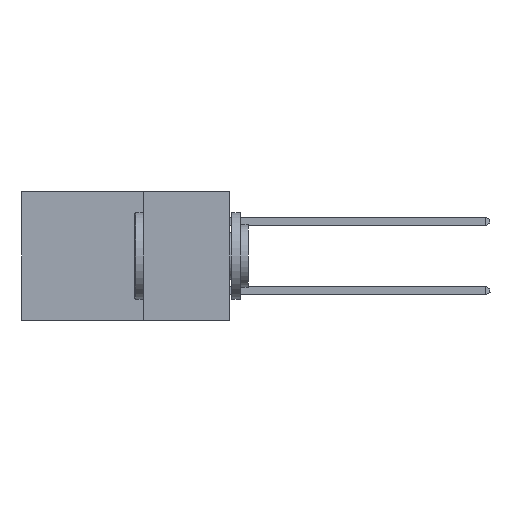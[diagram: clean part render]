
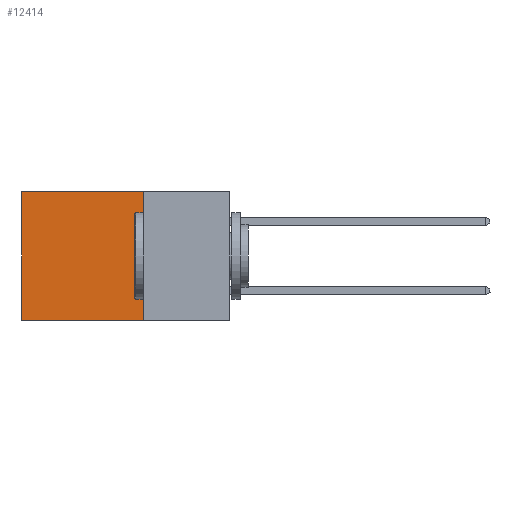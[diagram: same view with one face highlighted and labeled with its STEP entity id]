
A CAD part, left-side view. The second image highlights one B-rep face of the part: STEP entity #12414.
In plain terms, the highlighted planar face has unit normal (-1, 0, 0).
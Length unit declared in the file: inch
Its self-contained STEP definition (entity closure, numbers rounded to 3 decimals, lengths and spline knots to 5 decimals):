
#145 = AXIS2_PLACEMENT_3D ( 'NONE', #27502, #13374, #29830 ) ;
#390 = DIRECTION ( 'NONE',  ( 0., 1., 0. ) ) ;
#1108 = ORIENTED_EDGE ( 'NONE', *, *, #8051, .F. ) ;
#1260 = CARTESIAN_POINT ( 'NONE',  ( 0.298, 0.25, -0.37 ) ) ;
#1851 = CARTESIAN_POINT ( 'NONE',  ( 0.298, 0.25, -0.37 ) ) ;
#2516 = LINE ( 'NONE', #3339, #26216 ) ;
#2704 = VECTOR ( 'NONE', #30235, 39.37008 ) ;
#3339 = CARTESIAN_POINT ( 'NONE',  ( 0.298, 0.25, 0. ) ) ;
#3386 = FACE_OUTER_BOUND ( 'NONE', #28987, .T. ) ;
#5397 = CARTESIAN_POINT ( 'NONE',  ( 0.298, 0.6, 0. ) ) ;
#7564 = EDGE_CURVE ( 'NONE', #11516, #7725, #20928, .T. ) ;
#7725 = VERTEX_POINT ( 'NONE', #16689 ) ;
#8051 = EDGE_CURVE ( 'NONE', #11173, #20440, #2516, .T. ) ;
#8615 = PLANE ( 'NONE',  #145 ) ;
#10556 = DIRECTION ( 'NONE',  ( 0., 0., -1. ) ) ;
#10692 = EDGE_CURVE ( 'NONE', #11173, #11516, #22455, .T. ) ;
#11173 = VERTEX_POINT ( 'NONE', #16038 ) ;
#11516 = VERTEX_POINT ( 'NONE', #5397 ) ;
#12100 = LINE ( 'NONE', #1851, #27944 ) ;
#12414 = ADVANCED_FACE ( 'NONE', ( #3386 ), #8615, .F. ) ;
#13374 = DIRECTION ( 'NONE',  ( 1., 0., 0. ) ) ;
#13763 = CARTESIAN_POINT ( 'NONE',  ( 0.298, 0.6, 0. ) ) ;
#14284 = CARTESIAN_POINT ( 'NONE',  ( 0.298, 0.25, 0. ) ) ;
#14855 = ORIENTED_EDGE ( 'NONE', *, *, #16173, .F. ) ;
#16038 = CARTESIAN_POINT ( 'NONE',  ( 0.298, 0.25, 0. ) ) ;
#16127 = DIRECTION ( 'NONE',  ( 0., 1., 0. ) ) ;
#16173 = EDGE_CURVE ( 'NONE', #20440, #7725, #12100, .T. ) ;
#16689 = CARTESIAN_POINT ( 'NONE',  ( 0.298, 0.6, -0.37 ) ) ;
#20440 = VERTEX_POINT ( 'NONE', #1260 ) ;
#20928 = LINE ( 'NONE', #13763, #2704 ) ;
#21581 = ORIENTED_EDGE ( 'NONE', *, *, #10692, .T. ) ;
#21728 = VECTOR ( 'NONE', #390, 39.37008 ) ;
#22455 = LINE ( 'NONE', #14284, #21728 ) ;
#26216 = VECTOR ( 'NONE', #10556, 39.37008 ) ;
#26501 = ORIENTED_EDGE ( 'NONE', *, *, #7564, .T. ) ;
#27502 = CARTESIAN_POINT ( 'NONE',  ( 0.298, 0.25, 0. ) ) ;
#27944 = VECTOR ( 'NONE', #16127, 39.37008 ) ;
#28987 = EDGE_LOOP ( 'NONE', ( #26501, #14855, #1108, #21581 ) ) ;
#29830 = DIRECTION ( 'NONE',  ( 0., 0., -1. ) ) ;
#30235 = DIRECTION ( 'NONE',  ( 0., 0., -1. ) ) ;
